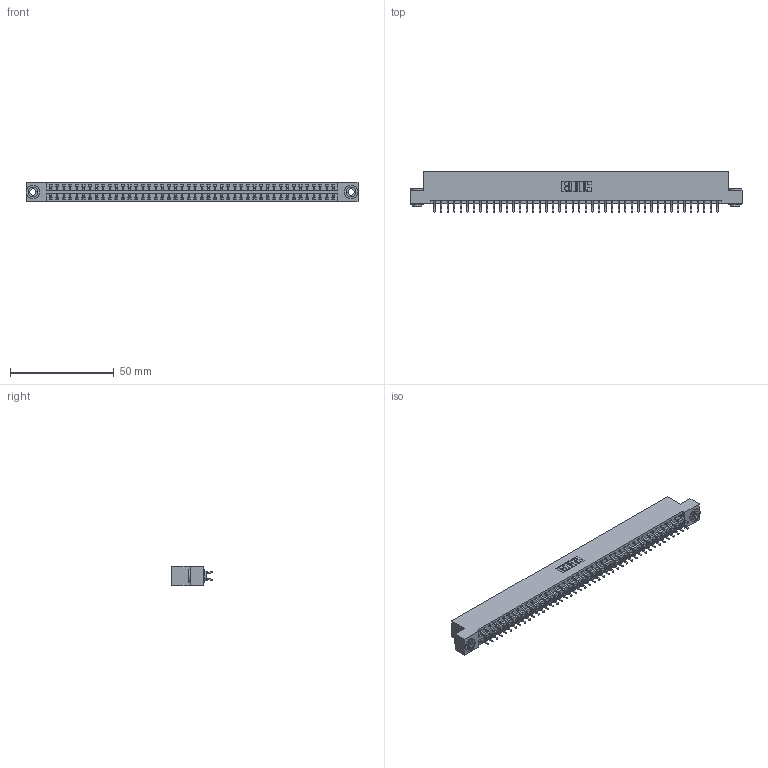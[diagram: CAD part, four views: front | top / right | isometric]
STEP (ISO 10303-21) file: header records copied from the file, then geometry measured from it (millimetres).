
FILE_DESCRIPTION (( 'STEP AP203' ), '1' );
FILE_NAME ('396-088-556-203.STEP', '2018-09-10T06:35:25', ( '' ), ( '' ), 'SwSTEP 2.0', 'SolidWorks 2016', '' );
FILE_SCHEMA (( 'CONFIG_CONTROL_DESIGN' ));
Length unit declared in the file: inch
Products named in the file (4): 346 Part_Flush Mounting Lugs - 0.156 Dia-TH; 345-292-001_556 Tail; 345-250-002_345-250-002-102; 396-088-556-203
Assembly tree (91 placements, depth 2):
  396-088-556-203
    346 Part_Flush Mounting Lugs - 0.156 Dia-TH
    345-292-001_556 Tail  x88
    345-250-002_345-250-002-102  x2
Bounding box: 160.27 x 19.57 x 9.4 mm (x, y, z)
Volume: 15660.1 mm3; surface area: 21689.8 mm2
Topology: 91 solids, 91 shells, 5264 faces, 15629 edges, 10298 vertices
Faces by surface type: plane 3518, cylinder 1738, cone 8
Entity records: 29316 total; most frequent: CARTESIAN_POINT 4819, ORIENTED_EDGE 4734, DIRECTION 4317, EDGE_CURVE 2367, VECTOR 2027, LINE 2027, VERTEX_POINT 1574, AXIS2_PLACEMENT_3D 1145
